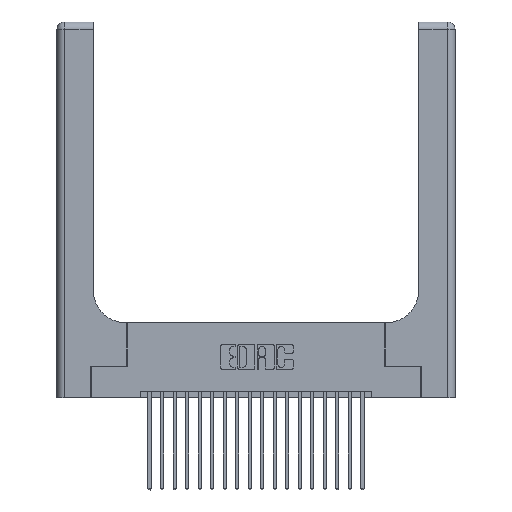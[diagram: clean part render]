
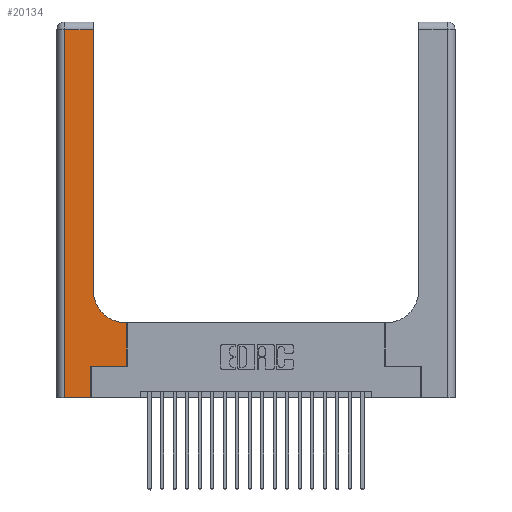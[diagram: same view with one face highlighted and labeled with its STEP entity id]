
A CAD part, top view. The second image highlights one B-rep face of the part: STEP entity #20134.
In plain terms, the highlighted planar face has unit normal (0, 0, 1).
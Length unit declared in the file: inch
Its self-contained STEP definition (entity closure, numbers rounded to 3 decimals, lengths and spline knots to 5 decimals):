
#337 = LINE ( 'NONE', #18655, #7429 ) ;
#1464 = VECTOR ( 'NONE', #5194, 39.37008 ) ;
#1520 = CARTESIAN_POINT ( 'NONE',  ( 0.06, 2.94, 0.37 ) ) ;
#2011 = CARTESIAN_POINT ( 'NONE',  ( 0.269, 0., 0.37 ) ) ;
#2042 = LINE ( 'NONE', #5385, #6100 ) ;
#2053 = AXIS2_PLACEMENT_3D ( 'NONE', #18231, #7848, #9674 ) ;
#2243 = VECTOR ( 'NONE', #14647, 39.37008 ) ;
#2537 = LINE ( 'NONE', #7172, #1464 ) ;
#2638 = CARTESIAN_POINT ( 'NONE',  ( 0.5585, 0.25, 0.37 ) ) ;
#3506 = CARTESIAN_POINT ( 'NONE',  ( 0.5585, 0.6, 0.37 ) ) ;
#3911 = VECTOR ( 'NONE', #13460, 39.37008 ) ;
#4104 = ORIENTED_EDGE ( 'NONE', *, *, #21693, .T. ) ;
#4499 = VERTEX_POINT ( 'NONE', #17458 ) ;
#4635 = LINE ( 'NONE', #2638, #8188 ) ;
#5194 = DIRECTION ( 'NONE',  ( 1., 0., 0. ) ) ;
#5304 = EDGE_CURVE ( 'NONE', #17982, #21083, #2042, .T. ) ;
#5312 = CARTESIAN_POINT ( 'NONE',  ( 0.2915, 2.94, 0.37 ) ) ;
#5314 = ORIENTED_EDGE ( 'NONE', *, *, #5639, .T. ) ;
#5353 = LINE ( 'NONE', #10277, #11944 ) ;
#5385 = CARTESIAN_POINT ( 'NONE',  ( 0.06, 3., 0.37 ) ) ;
#5639 = EDGE_CURVE ( 'NONE', #21083, #19963, #14496, .T. ) ;
#6033 = LINE ( 'NONE', #11661, #15314 ) ;
#6100 = VECTOR ( 'NONE', #15599, 39.37008 ) ;
#6314 = LINE ( 'NONE', #19560, #2243 ) ;
#7172 = CARTESIAN_POINT ( 'NONE',  ( 0.269, 0.25, 0.37 ) ) ;
#7429 = VECTOR ( 'NONE', #9943, 39.37008 ) ;
#7468 = CARTESIAN_POINT ( 'NONE',  ( 0.06, 0., 0.37 ) ) ;
#7823 = CARTESIAN_POINT ( 'NONE',  ( 0.2915, 0.85, 0.37 ) ) ;
#7848 = DIRECTION ( 'NONE',  ( 0., 0., -1. ) ) ;
#7904 = EDGE_CURVE ( 'NONE', #18803, #20509, #4635, .T. ) ;
#8188 = VECTOR ( 'NONE', #20141, 39.37008 ) ;
#8429 = ORIENTED_EDGE ( 'NONE', *, *, #10579, .T. ) ;
#9642 = VERTEX_POINT ( 'NONE', #11447 ) ;
#9674 = DIRECTION ( 'NONE',  ( 1., 0., 0. ) ) ;
#9943 = DIRECTION ( 'NONE',  ( -1., 0., 0. ) ) ;
#10277 = CARTESIAN_POINT ( 'NONE',  ( 0.2915, 3., 0.37 ) ) ;
#10579 = EDGE_CURVE ( 'NONE', #13605, #15589, #5353, .T. ) ;
#10990 = CARTESIAN_POINT ( 'NONE',  ( 0., 3., 0.37 ) ) ;
#11036 = EDGE_CURVE ( 'NONE', #15589, #17982, #337, .T. ) ;
#11235 = EDGE_CURVE ( 'NONE', #4499, #18803, #2537, .T. ) ;
#11447 = CARTESIAN_POINT ( 'NONE',  ( 0.5415, 0.6, 0.37 ) ) ;
#11516 = EDGE_CURVE ( 'NONE', #19963, #4499, #6033, .T. ) ;
#11661 = CARTESIAN_POINT ( 'NONE',  ( 0.269, 0., 0.37 ) ) ;
#11944 = VECTOR ( 'NONE', #12040, 39.37008 ) ;
#12040 = DIRECTION ( 'NONE',  ( 0., 1., 0. ) ) ;
#12093 = EDGE_LOOP ( 'NONE', ( #8429, #21724, #21433, #5314, #13872, #13493, #16273, #4104, #20295 ) ) ;
#13460 = DIRECTION ( 'NONE',  ( 1., 0., 0. ) ) ;
#13493 = ORIENTED_EDGE ( 'NONE', *, *, #11235, .T. ) ;
#13605 = VERTEX_POINT ( 'NONE', #7823 ) ;
#13872 = ORIENTED_EDGE ( 'NONE', *, *, #11516, .T. ) ;
#14496 = LINE ( 'NONE', #20244, #3911 ) ;
#14647 = DIRECTION ( 'NONE',  ( -1., 0., 0. ) ) ;
#14805 = EDGE_CURVE ( 'NONE', #9642, #13605, #16277, .T. ) ;
#14890 = DIRECTION ( 'NONE',  ( 0., 1., 0. ) ) ;
#15314 = VECTOR ( 'NONE', #14890, 39.37008 ) ;
#15589 = VERTEX_POINT ( 'NONE', #5312 ) ;
#15599 = DIRECTION ( 'NONE',  ( 0., -1., 0. ) ) ;
#16273 = ORIENTED_EDGE ( 'NONE', *, *, #7904, .T. ) ;
#16277 = CIRCLE ( 'NONE', #2053, 0.25 ) ;
#16431 = DIRECTION ( 'NONE',  ( 0., 0., -1. ) ) ;
#17208 = CARTESIAN_POINT ( 'NONE',  ( 0.5585, 0.25, 0.37 ) ) ;
#17407 = AXIS2_PLACEMENT_3D ( 'NONE', #10990, #16431, #18015 ) ;
#17458 = CARTESIAN_POINT ( 'NONE',  ( 0.269, 0.25, 0.37 ) ) ;
#17982 = VERTEX_POINT ( 'NONE', #1520 ) ;
#18015 = DIRECTION ( 'NONE',  ( -1., 0., 0. ) ) ;
#18231 = CARTESIAN_POINT ( 'NONE',  ( 0.5415, 0.85, 0.37 ) ) ;
#18234 = PLANE ( 'NONE',  #17407 ) ;
#18655 = CARTESIAN_POINT ( 'NONE',  ( 0., 2.94, 0.37 ) ) ;
#18803 = VERTEX_POINT ( 'NONE', #17208 ) ;
#19560 = CARTESIAN_POINT ( 'NONE',  ( 0.2915, 0.6, 0.37 ) ) ;
#19963 = VERTEX_POINT ( 'NONE', #2011 ) ;
#20134 = ADVANCED_FACE ( 'NONE', ( #20849 ), #18234, .F. ) ;
#20141 = DIRECTION ( 'NONE',  ( 0., 1., 0. ) ) ;
#20244 = CARTESIAN_POINT ( 'NONE',  ( 0., 0., 0.37 ) ) ;
#20295 = ORIENTED_EDGE ( 'NONE', *, *, #14805, .T. ) ;
#20509 = VERTEX_POINT ( 'NONE', #3506 ) ;
#20849 = FACE_OUTER_BOUND ( 'NONE', #12093, .T. ) ;
#21083 = VERTEX_POINT ( 'NONE', #7468 ) ;
#21433 = ORIENTED_EDGE ( 'NONE', *, *, #5304, .T. ) ;
#21693 = EDGE_CURVE ( 'NONE', #20509, #9642, #6314, .T. ) ;
#21724 = ORIENTED_EDGE ( 'NONE', *, *, #11036, .T. ) ;
